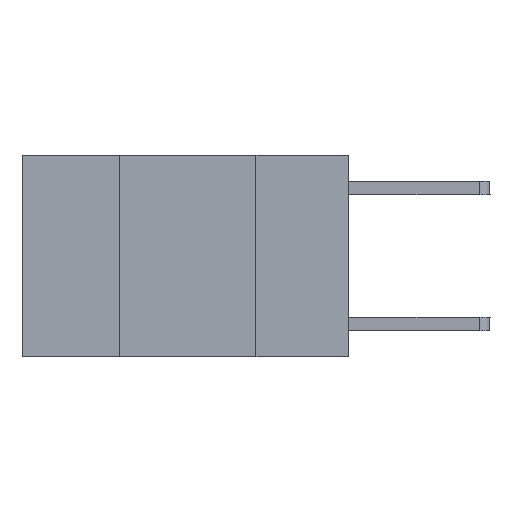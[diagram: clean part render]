
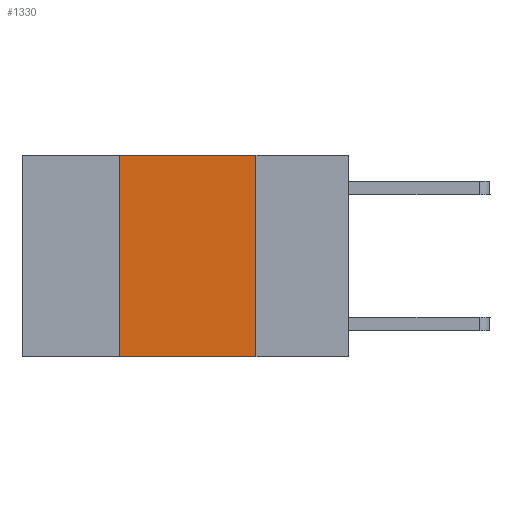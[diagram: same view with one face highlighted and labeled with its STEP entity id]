
A CAD part, left-side view. The second image highlights one B-rep face of the part: STEP entity #1330.
In plain terms, the highlighted planar face has unit normal (-1, 0, 0).
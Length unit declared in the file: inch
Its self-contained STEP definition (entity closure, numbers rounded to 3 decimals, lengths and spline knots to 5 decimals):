
#347 = DIRECTION ( 'NONE',  ( 0., 0., -1. ) ) ;
#397 = LINE ( 'NONE', #9381, #10004 ) ;
#1330 = ADVANCED_FACE ( 'NONE', ( #8715 ), #5989, .F. ) ;
#1801 = EDGE_CURVE ( 'NONE', #6382, #3830, #397, .T. ) ;
#1810 = EDGE_LOOP ( 'NONE', ( #8011, #5913, #2057, #5269 ) ) ;
#1947 = DIRECTION ( 'NONE',  ( 1., 0., 0. ) ) ;
#2057 = ORIENTED_EDGE ( 'NONE', *, *, #10058, .F. ) ;
#2155 = AXIS2_PLACEMENT_3D ( 'NONE', #9377, #1947, #7011 ) ;
#2224 = LINE ( 'NONE', #8980, #7046 ) ;
#2275 = EDGE_CURVE ( 'NONE', #6867, #3830, #9448, .T. ) ;
#3715 = CARTESIAN_POINT ( 'NONE',  ( 0., 0.42, -0.37 ) ) ;
#3830 = VERTEX_POINT ( 'NONE', #4221 ) ;
#4221 = CARTESIAN_POINT ( 'NONE',  ( 0., 0.17, -0.37 ) ) ;
#5087 = VECTOR ( 'NONE', #8861, 39.37008 ) ;
#5269 = ORIENTED_EDGE ( 'NONE', *, *, #2275, .T. ) ;
#5794 = EDGE_CURVE ( 'NONE', #9976, #6382, #2224, .T. ) ;
#5816 = CARTESIAN_POINT ( 'NONE',  ( 0., 0.17, 0. ) ) ;
#5913 = ORIENTED_EDGE ( 'NONE', *, *, #5794, .F. ) ;
#5989 = PLANE ( 'NONE',  #2155 ) ;
#6259 = DIRECTION ( 'NONE',  ( 0., 0., 1. ) ) ;
#6363 = DIRECTION ( 'NONE',  ( 0., -1., 0. ) ) ;
#6372 = CARTESIAN_POINT ( 'NONE',  ( 0., 0.42, 0. ) ) ;
#6382 = VERTEX_POINT ( 'NONE', #5816 ) ;
#6867 = VERTEX_POINT ( 'NONE', #3715 ) ;
#7011 = DIRECTION ( 'NONE',  ( 0., 0., -1. ) ) ;
#7046 = VECTOR ( 'NONE', #6363, 39.37008 ) ;
#7595 = CARTESIAN_POINT ( 'NONE',  ( 0., 0.42, 0. ) ) ;
#8011 = ORIENTED_EDGE ( 'NONE', *, *, #1801, .F. ) ;
#8715 = FACE_OUTER_BOUND ( 'NONE', #1810, .T. ) ;
#8861 = DIRECTION ( 'NONE',  ( 0., -1., 0. ) ) ;
#8980 = CARTESIAN_POINT ( 'NONE',  ( 0., 0.6, 0. ) ) ;
#9377 = CARTESIAN_POINT ( 'NONE',  ( 0., 0.6, 0. ) ) ;
#9381 = CARTESIAN_POINT ( 'NONE',  ( 0., 0.17, 0. ) ) ;
#9448 = LINE ( 'NONE', #10144, #5087 ) ;
#9976 = VERTEX_POINT ( 'NONE', #7595 ) ;
#10004 = VECTOR ( 'NONE', #347, 39.37008 ) ;
#10058 = EDGE_CURVE ( 'NONE', #6867, #9976, #10415, .T. ) ;
#10144 = CARTESIAN_POINT ( 'NONE',  ( 0., 0.6, -0.37 ) ) ;
#10415 = LINE ( 'NONE', #6372, #10574 ) ;
#10574 = VECTOR ( 'NONE', #6259, 39.37008 ) ;
